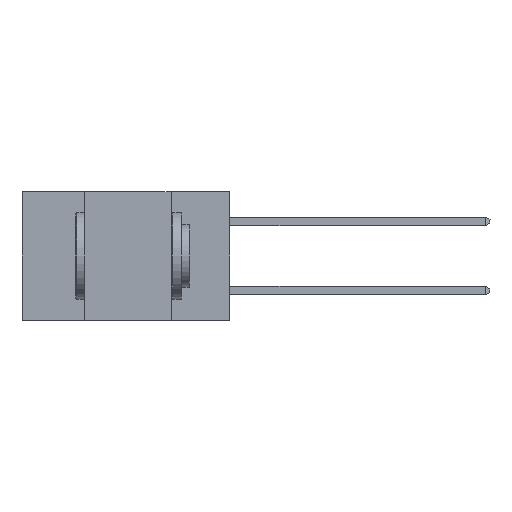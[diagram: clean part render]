
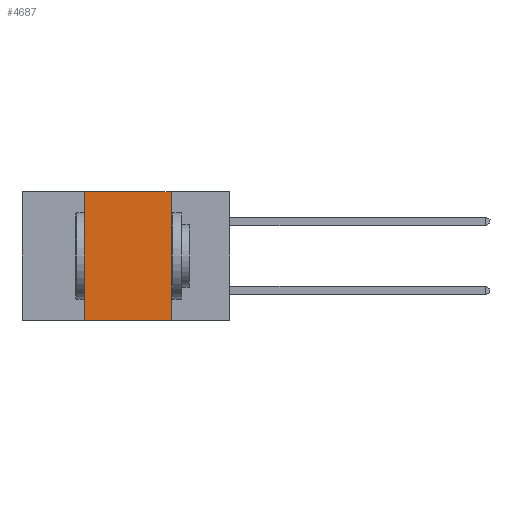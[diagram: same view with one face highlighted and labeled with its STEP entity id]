
A CAD part, left-side view. The second image highlights one B-rep face of the part: STEP entity #4687.
In plain terms, the highlighted planar face has unit normal (-1, 0, 0).
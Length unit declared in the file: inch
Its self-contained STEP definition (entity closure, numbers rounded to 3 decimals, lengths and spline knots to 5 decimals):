
#238 = DIRECTION ( 'NONE',  ( 0., -1., 0. ) ) ;
#1016 = EDGE_CURVE ( 'NONE', #3087, #1376, #8055, .T. ) ;
#1170 = DIRECTION ( 'NONE',  ( 0., -1., 0. ) ) ;
#1179 = VECTOR ( 'NONE', #10966, 39.37008 ) ;
#1376 = VERTEX_POINT ( 'NONE', #8602 ) ;
#1963 = AXIS2_PLACEMENT_3D ( 'NONE', #10540, #9721, #11460 ) ;
#2107 = VERTEX_POINT ( 'NONE', #9103 ) ;
#2133 = VECTOR ( 'NONE', #1170, 39.37008 ) ;
#2329 = ORIENTED_EDGE ( 'NONE', *, *, #6738, .T. ) ;
#2397 = DIRECTION ( 'NONE',  ( 0., 0., -1. ) ) ;
#2552 = FACE_OUTER_BOUND ( 'NONE', #11375, .T. ) ;
#2852 = CARTESIAN_POINT ( 'NONE',  ( 0., 0.17, 0. ) ) ;
#2893 = VERTEX_POINT ( 'NONE', #9676 ) ;
#3087 = VERTEX_POINT ( 'NONE', #2852 ) ;
#3294 = VECTOR ( 'NONE', #238, 39.37008 ) ;
#3746 = VECTOR ( 'NONE', #2397, 39.37008 ) ;
#3924 = LINE ( 'NONE', #7410, #3294 ) ;
#4687 = ADVANCED_FACE ( 'NONE', ( #2552 ), #9834, .F. ) ;
#4918 = LINE ( 'NONE', #11153, #2133 ) ;
#6738 = EDGE_CURVE ( 'NONE', #2893, #1376, #4918, .T. ) ;
#6752 = EDGE_CURVE ( 'NONE', #2107, #3087, #3924, .T. ) ;
#7109 = EDGE_CURVE ( 'NONE', #2893, #2107, #10795, .T. ) ;
#7410 = CARTESIAN_POINT ( 'NONE',  ( 0., 0.6, 0. ) ) ;
#7576 = ORIENTED_EDGE ( 'NONE', *, *, #1016, .F. ) ;
#8055 = LINE ( 'NONE', #9742, #3746 ) ;
#8266 = ORIENTED_EDGE ( 'NONE', *, *, #6752, .F. ) ;
#8602 = CARTESIAN_POINT ( 'NONE',  ( 0., 0.17, -0.37 ) ) ;
#9103 = CARTESIAN_POINT ( 'NONE',  ( 0., 0.42, 0. ) ) ;
#9676 = CARTESIAN_POINT ( 'NONE',  ( 0., 0.42, -0.37 ) ) ;
#9721 = DIRECTION ( 'NONE',  ( 1., 0., 0. ) ) ;
#9742 = CARTESIAN_POINT ( 'NONE',  ( 0., 0.17, -0.37 ) ) ;
#9834 = PLANE ( 'NONE',  #1963 ) ;
#9930 = CARTESIAN_POINT ( 'NONE',  ( 0., 0.42, -0.37 ) ) ;
#10540 = CARTESIAN_POINT ( 'NONE',  ( 0., 0.6, 0. ) ) ;
#10795 = LINE ( 'NONE', #9930, #1179 ) ;
#10966 = DIRECTION ( 'NONE',  ( 0., 0., 1. ) ) ;
#11153 = CARTESIAN_POINT ( 'NONE',  ( 0., 0.6, -0.37 ) ) ;
#11375 = EDGE_LOOP ( 'NONE', ( #7576, #8266, #11544, #2329 ) ) ;
#11460 = DIRECTION ( 'NONE',  ( 0., 0., -1. ) ) ;
#11544 = ORIENTED_EDGE ( 'NONE', *, *, #7109, .F. ) ;
